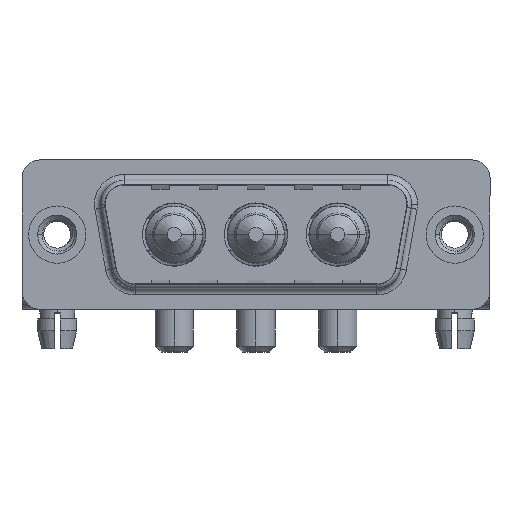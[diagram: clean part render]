
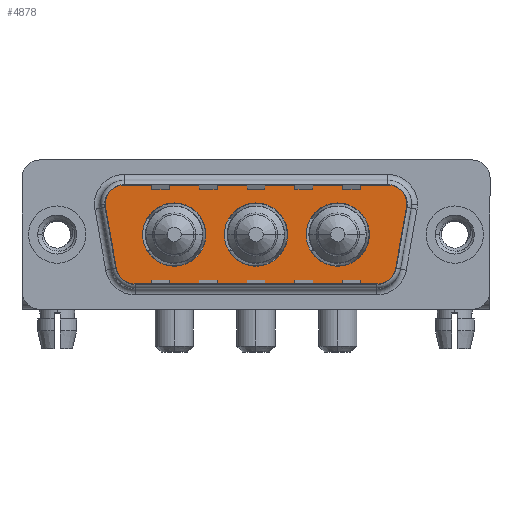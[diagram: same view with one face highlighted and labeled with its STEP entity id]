
A CAD part, top view. The second image highlights one B-rep face of the part: STEP entity #4878.
In plain terms, the highlighted planar face has unit normal (0, 0, 1).
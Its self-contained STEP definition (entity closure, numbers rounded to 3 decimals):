
#16 = CARTESIAN_POINT ( 'NONE',  ( 9.8, 0., 0. ) ) ;
#54 = DIRECTION ( 'NONE',  ( -1., 0., 0. ) ) ;
#66 = DIRECTION ( 'NONE',  ( 0., 0., 1. ) ) ;
#393 = CARTESIAN_POINT ( 'NONE',  ( 26.15, 0., 0. ) ) ;
#499 = VERTEX_POINT ( 'NONE', #7806 ) ;
#688 = ORIENTED_EDGE ( 'NONE', *, *, #8301, .F. ) ;
#756 = CARTESIAN_POINT ( 'NONE',  ( 23.5, 0., 0. ) ) ;
#792 = CARTESIAN_POINT ( 'NONE',  ( 16.65, 0., 0. ) ) ;
#837 = DIRECTION ( 'NONE',  ( 1., 0., 0. ) ) ;
#852 = VERTEX_POINT ( 'NONE', #14662 ) ;
#919 = CARTESIAN_POINT ( 'NONE',  ( 6.434, -4.9, 0. ) ) ;
#957 = DIRECTION ( 'NONE',  ( 1., 0., 0. ) ) ;
#1130 = EDGE_CURVE ( 'NONE', #7881, #7227, #6282, .T. ) ;
#1323 = CARTESIAN_POINT ( 'NONE',  ( 26.866, -2.9, 0. ) ) ;
#1327 = AXIS2_PLACEMENT_3D ( 'NONE', #1323, #10757, #4899 ) ;
#1435 = EDGE_CURVE ( 'NONE', #9563, #2224, #5068, .T. ) ;
#1592 = DIRECTION ( 'NONE',  ( 0., 0., 1. ) ) ;
#1765 = ORIENTED_EDGE ( 'NONE', *, *, #1435, .T. ) ;
#1767 = CIRCLE ( 'NONE', #6459, 2.65 ) ;
#1775 = DIRECTION ( 'NONE',  ( 0.174, -0.985, 0. ) ) ;
#2022 = CIRCLE ( 'NONE', #13125, 2.65 ) ;
#2224 = VERTEX_POINT ( 'NONE', #3875 ) ;
#2295 = EDGE_LOOP ( 'NONE', ( #2701, #7073 ) ) ;
#2529 = ORIENTED_EDGE ( 'NONE', *, *, #10464, .F. ) ;
#2697 = VERTEX_POINT ( 'NONE', #8917 ) ;
#2701 = ORIENTED_EDGE ( 'NONE', *, *, #11559, .F. ) ;
#2714 = CARTESIAN_POINT ( 'NONE',  ( 7.15, 0., 0. ) ) ;
#2755 = CARTESIAN_POINT ( 'NONE',  ( 16.65, 0., 0. ) ) ;
#2973 = AXIS2_PLACEMENT_3D ( 'NONE', #14886, #12571, #4542 ) ;
#3071 = FACE_OUTER_BOUND ( 'NONE', #4008, .T. ) ;
#3283 = AXIS2_PLACEMENT_3D ( 'NONE', #792, #5668, #957 ) ;
#3317 = AXIS2_PLACEMENT_3D ( 'NONE', #10624, #3671, #7376 ) ;
#3458 = VERTEX_POINT ( 'NONE', #13432 ) ;
#3671 = DIRECTION ( 'NONE',  ( 0., 0., 1. ) ) ;
#3708 = EDGE_CURVE ( 'NONE', #852, #499, #10494, .T. ) ;
#3859 = CARTESIAN_POINT ( 'NONE',  ( 9.8, 0., 0. ) ) ;
#3875 = CARTESIAN_POINT ( 'NONE',  ( 28.836, -3.247, 0. ) ) ;
#4008 = EDGE_LOOP ( 'NONE', ( #1765, #10070, #10731, #7475, #15023, #14294, #6467, #12129, #13136 ) ) ;
#4175 = VERTEX_POINT ( 'NONE', #10690 ) ;
#4542 = DIRECTION ( 'NONE',  ( -1., 0., 0. ) ) ;
#4682 = ORIENTED_EDGE ( 'NONE', *, *, #6022, .F. ) ;
#4728 = DIRECTION ( 'NONE',  ( 1., 0., 0. ) ) ;
#4762 = AXIS2_PLACEMENT_3D ( 'NONE', #2755, #6472, #8789 ) ;
#4775 = AXIS2_PLACEMENT_3D ( 'NONE', #14053, #66, #8256 ) ;
#4878 = ADVANCED_FACE ( 'NONE', ( #8717, #7569, #14822, #3071 ), #7798, .T. ) ;
#4899 = DIRECTION ( 'NONE',  ( 1., 0., 0. ) ) ;
#4951 = AXIS2_PLACEMENT_3D ( 'NONE', #10934, #1592, #12315 ) ;
#5068 = CIRCLE ( 'NONE', #14442, 2. ) ;
#5128 = VECTOR ( 'NONE', #54, 1000. ) ;
#5218 = VECTOR ( 'NONE', #9436, 1000. ) ;
#5414 = CARTESIAN_POINT ( 'NONE',  ( 3.441, 2.553, 0. ) ) ;
#5427 = AXIS2_PLACEMENT_3D ( 'NONE', #16, #14149, #4728 ) ;
#5548 = DIRECTION ( 'NONE',  ( 0.174, 0.985, 0. ) ) ;
#5668 = DIRECTION ( 'NONE',  ( 0., 0., 1. ) ) ;
#5744 = CARTESIAN_POINT ( 'NONE',  ( 26.866, -2.9, 0. ) ) ;
#6022 = EDGE_CURVE ( 'NONE', #6681, #2697, #1767, .T. ) ;
#6282 = CIRCLE ( 'NONE', #3317, 2. ) ;
#6459 = AXIS2_PLACEMENT_3D ( 'NONE', #11603, #15251, #10538 ) ;
#6467 = ORIENTED_EDGE ( 'NONE', *, *, #10845, .T. ) ;
#6472 = DIRECTION ( 'NONE',  ( 0., 0., 1. ) ) ;
#6609 = VERTEX_POINT ( 'NONE', #14373 ) ;
#6681 = VERTEX_POINT ( 'NONE', #393 ) ;
#6942 = EDGE_CURVE ( 'NONE', #499, #6944, #11440, .T. ) ;
#6944 = VERTEX_POINT ( 'NONE', #13201 ) ;
#7046 = AXIS2_PLACEMENT_3D ( 'NONE', #3859, #13423, #7473 ) ;
#7058 = EDGE_CURVE ( 'NONE', #6609, #3458, #11414, .T. ) ;
#7068 = EDGE_CURVE ( 'NONE', #4175, #14137, #7531, .T. ) ;
#7073 = ORIENTED_EDGE ( 'NONE', *, *, #7058, .F. ) ;
#7164 = EDGE_CURVE ( 'NONE', #2224, #9776, #7791, .T. ) ;
#7227 = VERTEX_POINT ( 'NONE', #919 ) ;
#7278 = EDGE_CURVE ( 'NONE', #9776, #13915, #8411, .T. ) ;
#7376 = DIRECTION ( 'NONE',  ( -1., 0., 0. ) ) ;
#7473 = DIRECTION ( 'NONE',  ( 1., 0., 0. ) ) ;
#7475 = ORIENTED_EDGE ( 'NONE', *, *, #7476, .T. ) ;
#7476 = EDGE_CURVE ( 'NONE', #13915, #852, #13302, .T. ) ;
#7531 = CIRCLE ( 'NONE', #7046, 2.65 ) ;
#7569 = FACE_BOUND ( 'NONE', #12686, .T. ) ;
#7725 = LINE ( 'NONE', #5414, #10921 ) ;
#7791 = LINE ( 'NONE', #13653, #11478 ) ;
#7798 = PLANE ( 'NONE',  #1327 ) ;
#7806 = CARTESIAN_POINT ( 'NONE',  ( 5.411, 4.9, 0. ) ) ;
#7881 = VERTEX_POINT ( 'NONE', #9532 ) ;
#8256 = DIRECTION ( 'NONE',  ( 1., 0., 0. ) ) ;
#8301 = EDGE_CURVE ( 'NONE', #14137, #4175, #12077, .T. ) ;
#8411 = CIRCLE ( 'NONE', #2973, 2. ) ;
#8717 = FACE_BOUND ( 'NONE', #2295, .T. ) ;
#8789 = DIRECTION ( 'NONE',  ( 1., 0., 0. ) ) ;
#8917 = CARTESIAN_POINT ( 'NONE',  ( 20.85, 0., 0. ) ) ;
#9436 = DIRECTION ( 'NONE',  ( 1., 0., 0. ) ) ;
#9532 = CARTESIAN_POINT ( 'NONE',  ( 4.464, -3.247, 0. ) ) ;
#9563 = VERTEX_POINT ( 'NONE', #12616 ) ;
#9705 = EDGE_CURVE ( 'NONE', #7227, #9563, #10670, .T. ) ;
#9776 = VERTEX_POINT ( 'NONE', #13935 ) ;
#9927 = CIRCLE ( 'NONE', #3283, 2.65 ) ;
#10070 = ORIENTED_EDGE ( 'NONE', *, *, #7164, .T. ) ;
#10451 = CARTESIAN_POINT ( 'NONE',  ( 6.434, -4.9, 0. ) ) ;
#10464 = EDGE_CURVE ( 'NONE', #2697, #6681, #2022, .T. ) ;
#10494 = LINE ( 'NONE', #14039, #5128 ) ;
#10538 = DIRECTION ( 'NONE',  ( 1., 0., 0. ) ) ;
#10624 = CARTESIAN_POINT ( 'NONE',  ( 6.434, -2.9, 0. ) ) ;
#10670 = LINE ( 'NONE', #10451, #5218 ) ;
#10690 = CARTESIAN_POINT ( 'NONE',  ( 12.45, 0., 0. ) ) ;
#10731 = ORIENTED_EDGE ( 'NONE', *, *, #7278, .T. ) ;
#10757 = DIRECTION ( 'NONE',  ( 0., 0., 1. ) ) ;
#10845 = EDGE_CURVE ( 'NONE', #6944, #7881, #7725, .T. ) ;
#10921 = VECTOR ( 'NONE', #1775, 1000. ) ;
#10934 = CARTESIAN_POINT ( 'NONE',  ( 27.889, 2.9, 0. ) ) ;
#11414 = CIRCLE ( 'NONE', #4762, 2.65 ) ;
#11440 = CIRCLE ( 'NONE', #4775, 2. ) ;
#11478 = VECTOR ( 'NONE', #5548, 1000. ) ;
#11542 = DIRECTION ( 'NONE',  ( 0., 0., 1. ) ) ;
#11559 = EDGE_CURVE ( 'NONE', #3458, #6609, #9927, .T. ) ;
#11603 = CARTESIAN_POINT ( 'NONE',  ( 23.5, 0., 0. ) ) ;
#12018 = EDGE_LOOP ( 'NONE', ( #12401, #688 ) ) ;
#12077 = CIRCLE ( 'NONE', #5427, 2.65 ) ;
#12129 = ORIENTED_EDGE ( 'NONE', *, *, #1130, .T. ) ;
#12315 = DIRECTION ( 'NONE',  ( -1., 0., 0. ) ) ;
#12401 = ORIENTED_EDGE ( 'NONE', *, *, #7068, .F. ) ;
#12571 = DIRECTION ( 'NONE',  ( 0., 0., 1. ) ) ;
#12616 = CARTESIAN_POINT ( 'NONE',  ( 26.866, -4.9, 0. ) ) ;
#12686 = EDGE_LOOP ( 'NONE', ( #4682, #2529 ) ) ;
#13125 = AXIS2_PLACEMENT_3D ( 'NONE', #756, #13582, #837 ) ;
#13136 = ORIENTED_EDGE ( 'NONE', *, *, #9705, .T. ) ;
#13201 = CARTESIAN_POINT ( 'NONE',  ( 3.441, 2.553, 0. ) ) ;
#13302 = CIRCLE ( 'NONE', #4951, 2. ) ;
#13423 = DIRECTION ( 'NONE',  ( 0., 0., 1. ) ) ;
#13432 = CARTESIAN_POINT ( 'NONE',  ( 19.3, 0., 0. ) ) ;
#13477 = CARTESIAN_POINT ( 'NONE',  ( 29.889, 2.9, 0. ) ) ;
#13582 = DIRECTION ( 'NONE',  ( 0., 0., 1. ) ) ;
#13653 = CARTESIAN_POINT ( 'NONE',  ( 29.859, 2.553, 0. ) ) ;
#13861 = DIRECTION ( 'NONE',  ( 1., 0., 0. ) ) ;
#13915 = VERTEX_POINT ( 'NONE', #13477 ) ;
#13935 = CARTESIAN_POINT ( 'NONE',  ( 29.859, 2.553, 0. ) ) ;
#14039 = CARTESIAN_POINT ( 'NONE',  ( 5.411, 4.9, 0. ) ) ;
#14053 = CARTESIAN_POINT ( 'NONE',  ( 5.411, 2.9, 0. ) ) ;
#14137 = VERTEX_POINT ( 'NONE', #2714 ) ;
#14149 = DIRECTION ( 'NONE',  ( 0., 0., 1. ) ) ;
#14294 = ORIENTED_EDGE ( 'NONE', *, *, #6942, .T. ) ;
#14373 = CARTESIAN_POINT ( 'NONE',  ( 14., 0., 0. ) ) ;
#14442 = AXIS2_PLACEMENT_3D ( 'NONE', #5744, #11542, #13861 ) ;
#14662 = CARTESIAN_POINT ( 'NONE',  ( 27.889, 4.9, 0. ) ) ;
#14822 = FACE_BOUND ( 'NONE', #12018, .T. ) ;
#14886 = CARTESIAN_POINT ( 'NONE',  ( 27.889, 2.9, 0. ) ) ;
#15023 = ORIENTED_EDGE ( 'NONE', *, *, #3708, .T. ) ;
#15251 = DIRECTION ( 'NONE',  ( 0., 0., 1. ) ) ;
